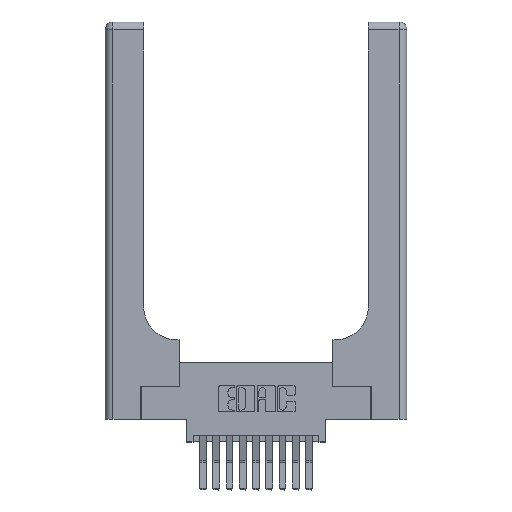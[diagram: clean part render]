
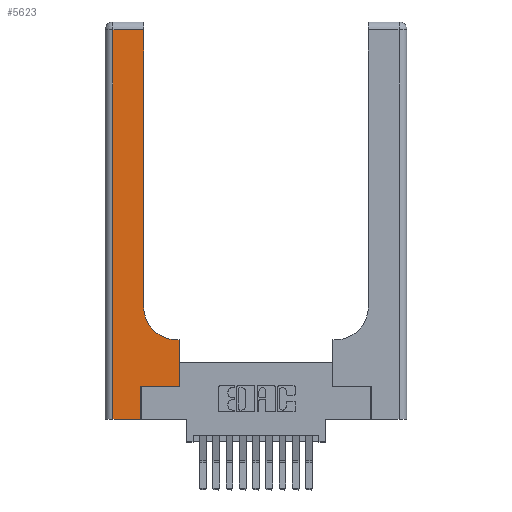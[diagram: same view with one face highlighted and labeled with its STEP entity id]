
A CAD part, top view. The second image highlights one B-rep face of the part: STEP entity #5623.
In plain terms, the highlighted planar face has unit normal (0, 0, 1).
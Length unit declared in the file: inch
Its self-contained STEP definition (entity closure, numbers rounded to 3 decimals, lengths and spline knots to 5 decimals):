
#25 = CARTESIAN_POINT ( 'NONE',  ( 0.06, 2.94, 0.37 ) ) ;
#327 = CARTESIAN_POINT ( 'NONE',  ( 0.269, 0., 0.37 ) ) ;
#467 = ORIENTED_EDGE ( 'NONE', *, *, #10667, .T. ) ;
#481 = CARTESIAN_POINT ( 'NONE',  ( 0.2915, 0.85, 0.37 ) ) ;
#785 = DIRECTION ( 'NONE',  ( 0., 0., -1. ) ) ;
#831 = ORIENTED_EDGE ( 'NONE', *, *, #8074, .T. ) ;
#1012 = VERTEX_POINT ( 'NONE', #9208 ) ;
#1471 = VERTEX_POINT ( 'NONE', #25 ) ;
#2503 = VECTOR ( 'NONE', #6335, 39.37008 ) ;
#2571 = CARTESIAN_POINT ( 'NONE',  ( 0.269, 0.25, 0.37 ) ) ;
#2991 = ORIENTED_EDGE ( 'NONE', *, *, #14242, .T. ) ;
#3152 = LINE ( 'NONE', #2571, #6671 ) ;
#3481 = EDGE_CURVE ( 'NONE', #13465, #5911, #7073, .T. ) ;
#3569 = VECTOR ( 'NONE', #15222, 39.37008 ) ;
#3859 = EDGE_LOOP ( 'NONE', ( #831, #7755, #9310, #6803, #11066, #14878, #9193, #2991, #467 ) ) ;
#3976 = PLANE ( 'NONE',  #12089 ) ;
#4913 = LINE ( 'NONE', #13123, #8708 ) ;
#5195 = DIRECTION ( 'NONE',  ( -1., 0., 0. ) ) ;
#5210 = LINE ( 'NONE', #16633, #14938 ) ;
#5251 = EDGE_CURVE ( 'NONE', #13673, #14341, #4913, .T. ) ;
#5496 = DIRECTION ( 'NONE',  ( 0., 1., 0. ) ) ;
#5623 = ADVANCED_FACE ( 'NONE', ( #13271 ), #3976, .F. ) ;
#5911 = VERTEX_POINT ( 'NONE', #327 ) ;
#6335 = DIRECTION ( 'NONE',  ( 0., 1., 0. ) ) ;
#6396 = VECTOR ( 'NONE', #11918, 39.37008 ) ;
#6671 = VECTOR ( 'NONE', #12936, 39.37008 ) ;
#6762 = CARTESIAN_POINT ( 'NONE',  ( 0.5585, 0.6, 0.37 ) ) ;
#6803 = ORIENTED_EDGE ( 'NONE', *, *, #3481, .T. ) ;
#7073 = LINE ( 'NONE', #8281, #13032 ) ;
#7594 = EDGE_CURVE ( 'NONE', #1012, #13673, #3152, .T. ) ;
#7642 = CARTESIAN_POINT ( 'NONE',  ( 0.2915, 3., 0.37 ) ) ;
#7755 = ORIENTED_EDGE ( 'NONE', *, *, #13554, .T. ) ;
#8074 = EDGE_CURVE ( 'NONE', #12120, #14350, #16380, .T. ) ;
#8281 = CARTESIAN_POINT ( 'NONE',  ( 0., 0., 0.37 ) ) ;
#8708 = VECTOR ( 'NONE', #5496, 39.37008 ) ;
#8781 = CARTESIAN_POINT ( 'NONE',  ( 0.5415, 0.85, 0.37 ) ) ;
#9169 = DIRECTION ( 'NONE',  ( -1., 0., 0. ) ) ;
#9193 = ORIENTED_EDGE ( 'NONE', *, *, #5251, .T. ) ;
#9208 = CARTESIAN_POINT ( 'NONE',  ( 0.269, 0.25, 0.37 ) ) ;
#9310 = ORIENTED_EDGE ( 'NONE', *, *, #9725, .T. ) ;
#9725 = EDGE_CURVE ( 'NONE', #1471, #13465, #10162, .T. ) ;
#9738 = CIRCLE ( 'NONE', #14147, 0.25 ) ;
#9971 = VERTEX_POINT ( 'NONE', #15053 ) ;
#10040 = DIRECTION ( 'NONE',  ( 1., 0., 0. ) ) ;
#10162 = LINE ( 'NONE', #15847, #6396 ) ;
#10591 = CARTESIAN_POINT ( 'NONE',  ( 0.2915, 2.94, 0.37 ) ) ;
#10667 = EDGE_CURVE ( 'NONE', #9971, #12120, #9738, .T. ) ;
#10780 = DIRECTION ( 'NONE',  ( 1., 0., 0. ) ) ;
#11014 = VECTOR ( 'NONE', #16770, 39.37008 ) ;
#11066 = ORIENTED_EDGE ( 'NONE', *, *, #12282, .T. ) ;
#11460 = LINE ( 'NONE', #15191, #2503 ) ;
#11918 = DIRECTION ( 'NONE',  ( 0., -1., 0. ) ) ;
#12089 = AXIS2_PLACEMENT_3D ( 'NONE', #15469, #16747, #9169 ) ;
#12120 = VERTEX_POINT ( 'NONE', #481 ) ;
#12282 = EDGE_CURVE ( 'NONE', #5911, #1012, #11460, .T. ) ;
#12936 = DIRECTION ( 'NONE',  ( 1., 0., 0. ) ) ;
#12973 = CARTESIAN_POINT ( 'NONE',  ( 0., 2.94, 0.37 ) ) ;
#13032 = VECTOR ( 'NONE', #10780, 39.37008 ) ;
#13123 = CARTESIAN_POINT ( 'NONE',  ( 0.5585, 0.25, 0.37 ) ) ;
#13271 = FACE_OUTER_BOUND ( 'NONE', #3859, .T. ) ;
#13465 = VERTEX_POINT ( 'NONE', #16226 ) ;
#13554 = EDGE_CURVE ( 'NONE', #14350, #1471, #14373, .T. ) ;
#13673 = VERTEX_POINT ( 'NONE', #15725 ) ;
#14147 = AXIS2_PLACEMENT_3D ( 'NONE', #8781, #785, #10040 ) ;
#14242 = EDGE_CURVE ( 'NONE', #14341, #9971, #5210, .T. ) ;
#14341 = VERTEX_POINT ( 'NONE', #6762 ) ;
#14350 = VERTEX_POINT ( 'NONE', #10591 ) ;
#14373 = LINE ( 'NONE', #12973, #11014 ) ;
#14878 = ORIENTED_EDGE ( 'NONE', *, *, #7594, .T. ) ;
#14938 = VECTOR ( 'NONE', #5195, 39.37008 ) ;
#15053 = CARTESIAN_POINT ( 'NONE',  ( 0.5415, 0.6, 0.37 ) ) ;
#15191 = CARTESIAN_POINT ( 'NONE',  ( 0.269, 0., 0.37 ) ) ;
#15222 = DIRECTION ( 'NONE',  ( 0., 1., 0. ) ) ;
#15469 = CARTESIAN_POINT ( 'NONE',  ( 0., 3., 0.37 ) ) ;
#15725 = CARTESIAN_POINT ( 'NONE',  ( 0.5585, 0.25, 0.37 ) ) ;
#15847 = CARTESIAN_POINT ( 'NONE',  ( 0.06, 3., 0.37 ) ) ;
#16226 = CARTESIAN_POINT ( 'NONE',  ( 0.06, 0., 0.37 ) ) ;
#16380 = LINE ( 'NONE', #7642, #3569 ) ;
#16633 = CARTESIAN_POINT ( 'NONE',  ( 0.2915, 0.6, 0.37 ) ) ;
#16747 = DIRECTION ( 'NONE',  ( 0., 0., -1. ) ) ;
#16770 = DIRECTION ( 'NONE',  ( -1., 0., 0. ) ) ;
